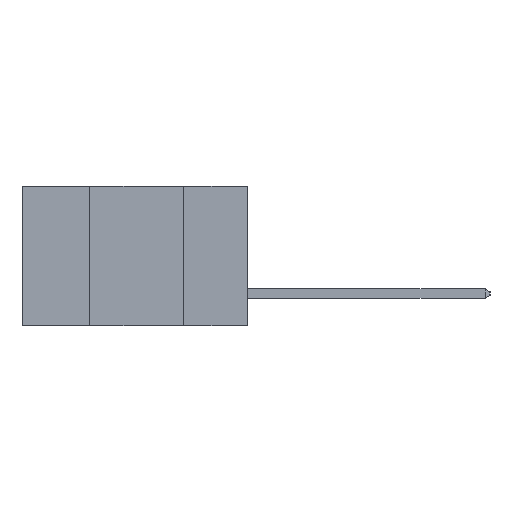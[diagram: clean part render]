
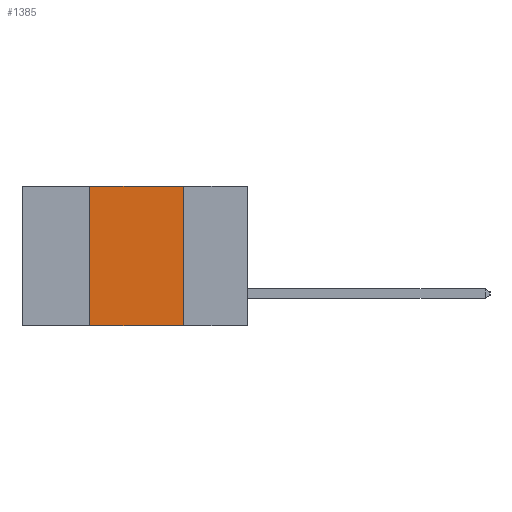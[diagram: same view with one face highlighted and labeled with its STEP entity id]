
A CAD part, left-side view. The second image highlights one B-rep face of the part: STEP entity #1385.
In plain terms, the highlighted planar face has unit normal (-1, 0, 0).
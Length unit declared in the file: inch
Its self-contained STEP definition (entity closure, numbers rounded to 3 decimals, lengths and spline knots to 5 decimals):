
#481 = VERTEX_POINT ( 'NONE', #13869 ) ;
#1385 = ADVANCED_FACE ( 'NONE', ( #15328 ), #8035, .F. ) ;
#1433 = LINE ( 'NONE', #12084, #10001 ) ;
#1812 = DIRECTION ( 'NONE',  ( 1., 0., 0. ) ) ;
#2184 = CARTESIAN_POINT ( 'NONE',  ( 0., 0.6, 0. ) ) ;
#2209 = CARTESIAN_POINT ( 'NONE',  ( 0., 0.42, -0.37 ) ) ;
#2514 = DIRECTION ( 'NONE',  ( 0., 0., -1. ) ) ;
#2819 = EDGE_CURVE ( 'NONE', #19531, #481, #4744, .T. ) ;
#3013 = LINE ( 'NONE', #16638, #12562 ) ;
#3082 = CARTESIAN_POINT ( 'NONE',  ( 0., 0.42, 0. ) ) ;
#3202 = CARTESIAN_POINT ( 'NONE',  ( 0., 0.17, -0.37 ) ) ;
#4744 = LINE ( 'NONE', #3202, #21256 ) ;
#6051 = VERTEX_POINT ( 'NONE', #2209 ) ;
#6757 = EDGE_CURVE ( 'NONE', #7349, #19531, #1433, .T. ) ;
#7349 = VERTEX_POINT ( 'NONE', #3082 ) ;
#8035 = PLANE ( 'NONE',  #20038 ) ;
#8965 = DIRECTION ( 'NONE',  ( 0., 0., -1. ) ) ;
#10001 = VECTOR ( 'NONE', #11868, 39.37008 ) ;
#10596 = DIRECTION ( 'NONE',  ( 0., 0., 1. ) ) ;
#10849 = CARTESIAN_POINT ( 'NONE',  ( 0., 0.42, -0.37 ) ) ;
#11087 = ORIENTED_EDGE ( 'NONE', *, *, #2819, .F. ) ;
#11868 = DIRECTION ( 'NONE',  ( 0., -1., 0. ) ) ;
#12084 = CARTESIAN_POINT ( 'NONE',  ( 0., 0.6, 0. ) ) ;
#12117 = ORIENTED_EDGE ( 'NONE', *, *, #16068, .F. ) ;
#12562 = VECTOR ( 'NONE', #21411, 39.37008 ) ;
#13869 = CARTESIAN_POINT ( 'NONE',  ( 0., 0.17, -0.37 ) ) ;
#15328 = FACE_OUTER_BOUND ( 'NONE', #20221, .T. ) ;
#15473 = ORIENTED_EDGE ( 'NONE', *, *, #6757, .F. ) ;
#16068 = EDGE_CURVE ( 'NONE', #6051, #7349, #16226, .T. ) ;
#16226 = LINE ( 'NONE', #10849, #16737 ) ;
#16497 = ORIENTED_EDGE ( 'NONE', *, *, #19719, .T. ) ;
#16638 = CARTESIAN_POINT ( 'NONE',  ( 0., 0.6, -0.37 ) ) ;
#16737 = VECTOR ( 'NONE', #10596, 39.37008 ) ;
#19389 = CARTESIAN_POINT ( 'NONE',  ( 0., 0.17, 0. ) ) ;
#19531 = VERTEX_POINT ( 'NONE', #19389 ) ;
#19719 = EDGE_CURVE ( 'NONE', #6051, #481, #3013, .T. ) ;
#20038 = AXIS2_PLACEMENT_3D ( 'NONE', #2184, #1812, #8965 ) ;
#20221 = EDGE_LOOP ( 'NONE', ( #11087, #15473, #12117, #16497 ) ) ;
#21256 = VECTOR ( 'NONE', #2514, 39.37008 ) ;
#21411 = DIRECTION ( 'NONE',  ( 0., -1., 0. ) ) ;
